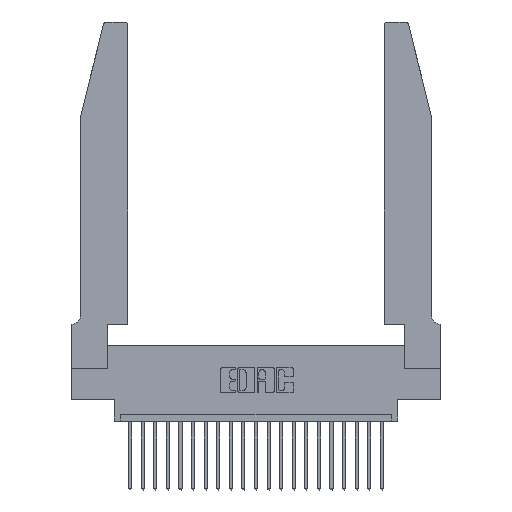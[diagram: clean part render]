
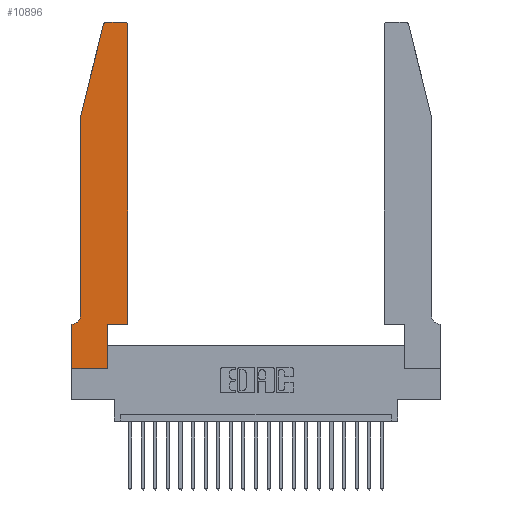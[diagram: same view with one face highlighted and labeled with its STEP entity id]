
A CAD part, top view. The second image highlights one B-rep face of the part: STEP entity #10896.
In plain terms, the highlighted planar face has unit normal (0, 0, 1).
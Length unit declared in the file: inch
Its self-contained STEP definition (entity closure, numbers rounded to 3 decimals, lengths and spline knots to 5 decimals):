
#654 = ORIENTED_EDGE ( 'NONE', *, *, #4985, .T. ) ;
#805 = DIRECTION ( 'NONE',  ( 0., -1., 0. ) ) ;
#872 = VERTEX_POINT ( 'NONE', #4174 ) ;
#1014 = VECTOR ( 'NONE', #22645, 39.37008 ) ;
#1073 = CARTESIAN_POINT ( 'NONE',  ( 0.2865, 0.35, 0.37 ) ) ;
#1158 = CIRCLE ( 'NONE', #11572, 0.03 ) ;
#1167 = VECTOR ( 'NONE', #6650, 39.37008 ) ;
#1194 = AXIS2_PLACEMENT_3D ( 'NONE', #10683, #5366, #18187 ) ;
#1370 = CARTESIAN_POINT ( 'NONE',  ( 0.4505, 0.35, 0.37 ) ) ;
#1482 = EDGE_CURVE ( 'NONE', #10830, #16190, #9807, .T. ) ;
#1686 = VERTEX_POINT ( 'NONE', #14237 ) ;
#1789 = EDGE_CURVE ( 'NONE', #16948, #1686, #16919, .T. ) ;
#2242 = AXIS2_PLACEMENT_3D ( 'NONE', #6412, #5571, #7638 ) ;
#2598 = EDGE_CURVE ( 'NONE', #1686, #16556, #22615, .T. ) ;
#2749 = CARTESIAN_POINT ( 'NONE',  ( 0.0755, 0.35, 0.37 ) ) ;
#3044 = DIRECTION ( 'NONE',  ( -1., 0., 0. ) ) ;
#3075 = DIRECTION ( 'NONE',  ( -1., 0., 0. ) ) ;
#3643 = VERTEX_POINT ( 'NONE', #12372 ) ;
#3869 = DIRECTION ( 'NONE',  ( -1., 0., 0. ) ) ;
#3970 = CARTESIAN_POINT ( 'NONE',  ( 0., 0., 0.37 ) ) ;
#4174 = CARTESIAN_POINT ( 'NONE',  ( 0.4205, 2.75, 0.37 ) ) ;
#4643 = ORIENTED_EDGE ( 'NONE', *, *, #1482, .T. ) ;
#4959 = DIRECTION ( 'NONE',  ( 0., 0., 1. ) ) ;
#4985 = EDGE_CURVE ( 'NONE', #3643, #12019, #1158, .T. ) ;
#5137 = ORIENTED_EDGE ( 'NONE', *, *, #11688, .T. ) ;
#5284 = EDGE_CURVE ( 'NONE', #12019, #6883, #16759, .T. ) ;
#5366 = DIRECTION ( 'NONE',  ( 0., 0., 1. ) ) ;
#5571 = DIRECTION ( 'NONE',  ( 0., 0., 1. ) ) ;
#5826 = DIRECTION ( 'NONE',  ( 0., 0., -1. ) ) ;
#5851 = LINE ( 'NONE', #15930, #21264 ) ;
#6268 = LINE ( 'NONE', #6411, #1167 ) ;
#6411 = CARTESIAN_POINT ( 'NONE',  ( 0.0755, 2., 0.37 ) ) ;
#6412 = CARTESIAN_POINT ( 'NONE',  ( 0., 0.35, 0.37 ) ) ;
#6467 = EDGE_CURVE ( 'NONE', #13408, #10830, #19018, .T. ) ;
#6650 = DIRECTION ( 'NONE',  ( 0., -1., 0. ) ) ;
#6883 = VERTEX_POINT ( 'NONE', #18463 ) ;
#6971 = ORIENTED_EDGE ( 'NONE', *, *, #10178, .T. ) ;
#7236 = ORIENTED_EDGE ( 'NONE', *, *, #11963, .T. ) ;
#7360 = ORIENTED_EDGE ( 'NONE', *, *, #12375, .T. ) ;
#7437 = ORIENTED_EDGE ( 'NONE', *, *, #6467, .T. ) ;
#7512 = EDGE_CURVE ( 'NONE', #872, #3643, #5851, .T. ) ;
#7638 = DIRECTION ( 'NONE',  ( 1., 0., 0. ) ) ;
#8028 = CARTESIAN_POINT ( 'NONE',  ( 0.4505, 0.35, 0.37 ) ) ;
#8034 = VERTEX_POINT ( 'NONE', #8051 ) ;
#8051 = CARTESIAN_POINT ( 'NONE',  ( 0.4505, 0.35, 0.37 ) ) ;
#8253 = DIRECTION ( 'NONE',  ( 1., 0., 0. ) ) ;
#8341 = ORIENTED_EDGE ( 'NONE', *, *, #1789, .T. ) ;
#8580 = DIRECTION ( 'NONE',  ( 0., 1., 0. ) ) ;
#9334 = CIRCLE ( 'NONE', #1194, 0.03 ) ;
#9807 = LINE ( 'NONE', #21062, #1014 ) ;
#10178 = EDGE_CURVE ( 'NONE', #8034, #14991, #22837, .T. ) ;
#10683 = CARTESIAN_POINT ( 'NONE',  ( 0.4205, 2.72, 0.37 ) ) ;
#10830 = VERTEX_POINT ( 'NONE', #19517 ) ;
#10896 = ADVANCED_FACE ( 'NONE', ( #22529 ), #13334, .T. ) ;
#10972 = CARTESIAN_POINT ( 'NONE',  ( 0.0755, 2., 0.37 ) ) ;
#11572 = AXIS2_PLACEMENT_3D ( 'NONE', #17610, #4959, #19538 ) ;
#11662 = ORIENTED_EDGE ( 'NONE', *, *, #5284, .T. ) ;
#11688 = EDGE_CURVE ( 'NONE', #6883, #16948, #6268, .T. ) ;
#11819 = CARTESIAN_POINT ( 'NONE',  ( 0., 0., 0.37 ) ) ;
#11963 = EDGE_CURVE ( 'NONE', #16190, #8034, #17072, .T. ) ;
#12019 = VERTEX_POINT ( 'NONE', #20738 ) ;
#12372 = CARTESIAN_POINT ( 'NONE',  ( 0.284, 2.75, 0.37 ) ) ;
#12375 = EDGE_CURVE ( 'NONE', #14991, #872, #9334, .T. ) ;
#12902 = VECTOR ( 'NONE', #3044, 39.37008 ) ;
#12969 = LINE ( 'NONE', #11819, #18990 ) ;
#13334 = PLANE ( 'NONE',  #2242 ) ;
#13408 = VERTEX_POINT ( 'NONE', #20549 ) ;
#13437 = ORIENTED_EDGE ( 'NONE', *, *, #7512, .T. ) ;
#14237 = CARTESIAN_POINT ( 'NONE',  ( 0.0055, 0.35, 0.37 ) ) ;
#14843 = DIRECTION ( 'NONE',  ( 1., 0., 0. ) ) ;
#14857 = VECTOR ( 'NONE', #8580, 39.37008 ) ;
#14991 = VERTEX_POINT ( 'NONE', #17489 ) ;
#15930 = CARTESIAN_POINT ( 'NONE',  ( 0.2605, 2.75, 0.37 ) ) ;
#15934 = CARTESIAN_POINT ( 'NONE',  ( 0., 0.35, 0.37 ) ) ;
#15977 = EDGE_LOOP ( 'NONE', ( #13437, #654, #11662, #5137, #8341, #23123, #20827, #7437, #4643, #7236, #6971, #7360 ) ) ;
#16162 = VECTOR ( 'NONE', #20269, 39.37008 ) ;
#16190 = VERTEX_POINT ( 'NONE', #1073 ) ;
#16432 = VECTOR ( 'NONE', #14843, 39.37008 ) ;
#16556 = VERTEX_POINT ( 'NONE', #15934 ) ;
#16759 = LINE ( 'NONE', #10972, #16162 ) ;
#16770 = VECTOR ( 'NONE', #8253, 39.37008 ) ;
#16919 = CIRCLE ( 'NONE', #20727, 0.07 ) ;
#16948 = VERTEX_POINT ( 'NONE', #17096 ) ;
#17072 = LINE ( 'NONE', #8028, #16770 ) ;
#17096 = CARTESIAN_POINT ( 'NONE',  ( 0.0755, 0.42, 0.37 ) ) ;
#17425 = EDGE_CURVE ( 'NONE', #16556, #13408, #12969, .T. ) ;
#17489 = CARTESIAN_POINT ( 'NONE',  ( 0.4505, 2.72, 0.37 ) ) ;
#17610 = CARTESIAN_POINT ( 'NONE',  ( 0.284, 2.72, 0.37 ) ) ;
#18187 = DIRECTION ( 'NONE',  ( 1., 0., 0. ) ) ;
#18463 = CARTESIAN_POINT ( 'NONE',  ( 0.0755, 2., 0.37 ) ) ;
#18990 = VECTOR ( 'NONE', #805, 39.37008 ) ;
#19018 = LINE ( 'NONE', #3970, #16432 ) ;
#19517 = CARTESIAN_POINT ( 'NONE',  ( 0.2865, 0., 0.37 ) ) ;
#19538 = DIRECTION ( 'NONE',  ( 1., 0., 0. ) ) ;
#20269 = DIRECTION ( 'NONE',  ( -0.239, -0.971, 0. ) ) ;
#20368 = CARTESIAN_POINT ( 'NONE',  ( 0.0055, 0.42, 0.37 ) ) ;
#20549 = CARTESIAN_POINT ( 'NONE',  ( 0., 0., 0.37 ) ) ;
#20727 = AXIS2_PLACEMENT_3D ( 'NONE', #20368, #5826, #3869 ) ;
#20738 = CARTESIAN_POINT ( 'NONE',  ( 0.25487, 2.72718, 0.37 ) ) ;
#20827 = ORIENTED_EDGE ( 'NONE', *, *, #17425, .T. ) ;
#21062 = CARTESIAN_POINT ( 'NONE',  ( 0.2865, 0.35, 0.37 ) ) ;
#21264 = VECTOR ( 'NONE', #3075, 39.37008 ) ;
#22529 = FACE_OUTER_BOUND ( 'NONE', #15977, .T. ) ;
#22615 = LINE ( 'NONE', #2749, #12902 ) ;
#22645 = DIRECTION ( 'NONE',  ( 0., 1., 0. ) ) ;
#22837 = LINE ( 'NONE', #1370, #14857 ) ;
#23123 = ORIENTED_EDGE ( 'NONE', *, *, #2598, .T. ) ;
